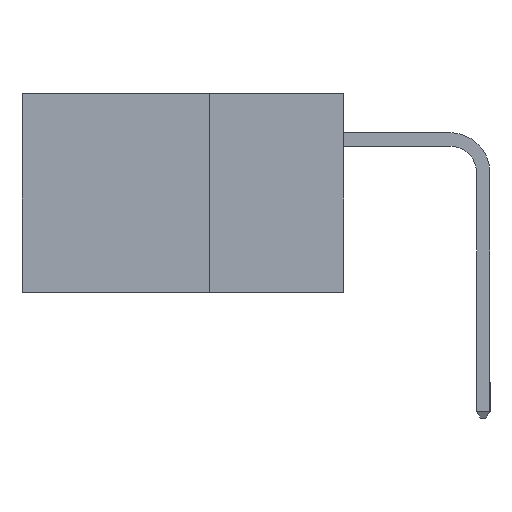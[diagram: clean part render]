
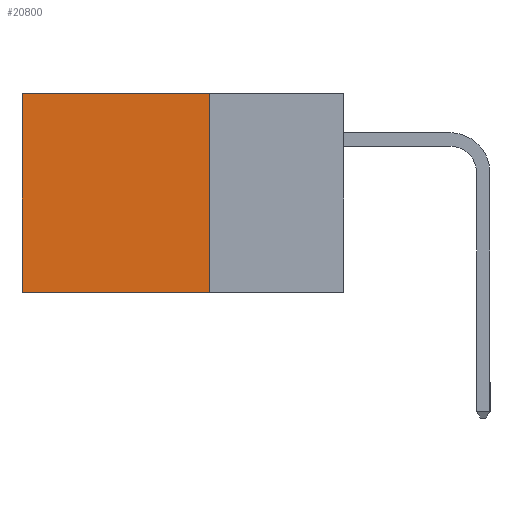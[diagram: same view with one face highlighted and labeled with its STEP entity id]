
A CAD part, left-side view. The second image highlights one B-rep face of the part: STEP entity #20800.
In plain terms, the highlighted planar face has unit normal (-1, 0, 0).
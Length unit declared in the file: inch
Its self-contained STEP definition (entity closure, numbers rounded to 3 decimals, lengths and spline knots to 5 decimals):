
#73 = EDGE_LOOP ( 'NONE', ( #11342, #20798, #19030, #23124 ) ) ;
#342 = EDGE_CURVE ( 'NONE', #14803, #5484, #6028, .T. ) ;
#836 = DIRECTION ( 'NONE',  ( 0., 1., 0. ) ) ;
#2907 = VERTEX_POINT ( 'NONE', #22389 ) ;
#3018 = VECTOR ( 'NONE', #14799, 39.37008 ) ;
#5078 = LINE ( 'NONE', #14912, #20273 ) ;
#5347 = FACE_OUTER_BOUND ( 'NONE', #73, .T. ) ;
#5484 = VERTEX_POINT ( 'NONE', #16605 ) ;
#5806 = CARTESIAN_POINT ( 'NONE',  ( 0.298, 0.25, -0.37 ) ) ;
#6028 = LINE ( 'NONE', #11311, #16628 ) ;
#6287 = DIRECTION ( 'NONE',  ( 0., 1., 0. ) ) ;
#7624 = CARTESIAN_POINT ( 'NONE',  ( 0.298, 0.25, 0. ) ) ;
#8397 = LINE ( 'NONE', #14716, #3018 ) ;
#9718 = DIRECTION ( 'NONE',  ( 1., 0., 0. ) ) ;
#11311 = CARTESIAN_POINT ( 'NONE',  ( 0.298, 0.25, -0.37 ) ) ;
#11342 = ORIENTED_EDGE ( 'NONE', *, *, #11773, .T. ) ;
#11773 = EDGE_CURVE ( 'NONE', #2907, #5484, #5078, .T. ) ;
#13642 = EDGE_CURVE ( 'NONE', #19906, #2907, #14681, .T. ) ;
#14270 = EDGE_CURVE ( 'NONE', #19906, #14803, #8397, .T. ) ;
#14681 = LINE ( 'NONE', #24627, #24441 ) ;
#14716 = CARTESIAN_POINT ( 'NONE',  ( 0.298, 0.25, 0. ) ) ;
#14799 = DIRECTION ( 'NONE',  ( 0., 0., -1. ) ) ;
#14803 = VERTEX_POINT ( 'NONE', #5806 ) ;
#14912 = CARTESIAN_POINT ( 'NONE',  ( 0.298, 0.6, 0. ) ) ;
#15399 = CARTESIAN_POINT ( 'NONE',  ( 0.298, 0.25, 0. ) ) ;
#16605 = CARTESIAN_POINT ( 'NONE',  ( 0.298, 0.6, -0.37 ) ) ;
#16628 = VECTOR ( 'NONE', #6287, 39.37008 ) ;
#16872 = DIRECTION ( 'NONE',  ( 0., 0., -1. ) ) ;
#19030 = ORIENTED_EDGE ( 'NONE', *, *, #14270, .F. ) ;
#19906 = VERTEX_POINT ( 'NONE', #15399 ) ;
#20273 = VECTOR ( 'NONE', #16872, 39.37008 ) ;
#20798 = ORIENTED_EDGE ( 'NONE', *, *, #342, .F. ) ;
#20800 = ADVANCED_FACE ( 'NONE', ( #5347 ), #21492, .F. ) ;
#21492 = PLANE ( 'NONE',  #24451 ) ;
#22389 = CARTESIAN_POINT ( 'NONE',  ( 0.298, 0.6, 0. ) ) ;
#23124 = ORIENTED_EDGE ( 'NONE', *, *, #13642, .T. ) ;
#23464 = DIRECTION ( 'NONE',  ( 0., 0., -1. ) ) ;
#24441 = VECTOR ( 'NONE', #836, 39.37008 ) ;
#24451 = AXIS2_PLACEMENT_3D ( 'NONE', #7624, #9718, #23464 ) ;
#24627 = CARTESIAN_POINT ( 'NONE',  ( 0.298, 0.25, 0. ) ) ;
